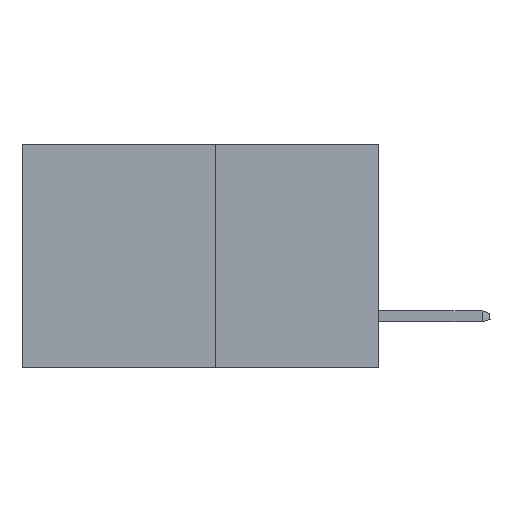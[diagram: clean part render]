
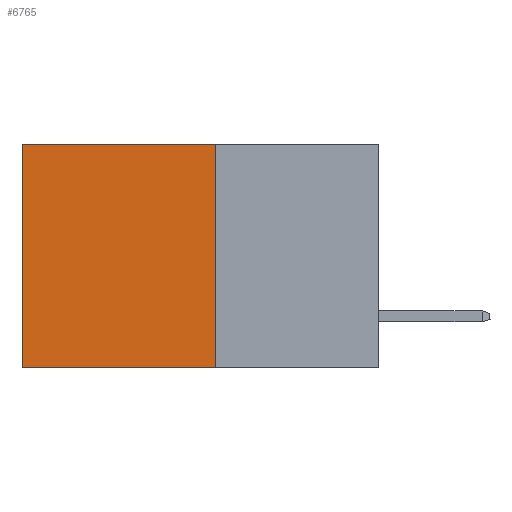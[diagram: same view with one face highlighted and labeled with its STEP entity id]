
A CAD part, left-side view. The second image highlights one B-rep face of the part: STEP entity #6765.
In plain terms, the highlighted planar face has unit normal (-1, 0, 0).
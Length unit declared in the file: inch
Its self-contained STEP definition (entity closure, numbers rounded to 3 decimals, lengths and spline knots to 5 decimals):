
#218 = ORIENTED_EDGE ( 'NONE', *, *, #3542, .T. ) ;
#1036 = LINE ( 'NONE', #17125, #4807 ) ;
#1118 = VERTEX_POINT ( 'NONE', #12207 ) ;
#1939 = EDGE_CURVE ( 'NONE', #14651, #1118, #13959, .T. ) ;
#2101 = ORIENTED_EDGE ( 'NONE', *, *, #7734, .T. ) ;
#2367 = DIRECTION ( 'NONE',  ( 0., 0., -1. ) ) ;
#3542 = EDGE_CURVE ( 'NONE', #18680, #8754, #1036, .T. ) ;
#3758 = ORIENTED_EDGE ( 'NONE', *, *, #1939, .F. ) ;
#4144 = VECTOR ( 'NONE', #14980, 39.37008 ) ;
#4807 = VECTOR ( 'NONE', #2367, 39.37008 ) ;
#5263 = CARTESIAN_POINT ( 'NONE',  ( 0.277, 0.27, -0.37 ) ) ;
#5290 = DIRECTION ( 'NONE',  ( 0., 1., 0. ) ) ;
#6765 = ADVANCED_FACE ( 'NONE', ( #9466 ), #14829, .F. ) ;
#7539 = CARTESIAN_POINT ( 'NONE',  ( 0.277, 0.27, -0.37 ) ) ;
#7734 = EDGE_CURVE ( 'NONE', #14651, #18680, #16158, .T. ) ;
#8754 = VERTEX_POINT ( 'NONE', #15843 ) ;
#9466 = FACE_OUTER_BOUND ( 'NONE', #19459, .T. ) ;
#9657 = CARTESIAN_POINT ( 'NONE',  ( 0.277, 0.27, -0.37 ) ) ;
#9986 = EDGE_CURVE ( 'NONE', #1118, #8754, #15811, .T. ) ;
#10418 = DIRECTION ( 'NONE',  ( 0., 0., -1. ) ) ;
#12207 = CARTESIAN_POINT ( 'NONE',  ( 0.277, 0.27, -0.37 ) ) ;
#12299 = VECTOR ( 'NONE', #5290, 39.37008 ) ;
#13959 = LINE ( 'NONE', #9657, #17522 ) ;
#14651 = VERTEX_POINT ( 'NONE', #15709 ) ;
#14829 = PLANE ( 'NONE',  #17242 ) ;
#14980 = DIRECTION ( 'NONE',  ( 0., 1., 0. ) ) ;
#15602 = CARTESIAN_POINT ( 'NONE',  ( 0.277, 0.27, 0. ) ) ;
#15709 = CARTESIAN_POINT ( 'NONE',  ( 0.277, 0.27, 0. ) ) ;
#15811 = LINE ( 'NONE', #5263, #12299 ) ;
#15843 = CARTESIAN_POINT ( 'NONE',  ( 0.277, 0.59, -0.37 ) ) ;
#16158 = LINE ( 'NONE', #15602, #4144 ) ;
#17007 = CARTESIAN_POINT ( 'NONE',  ( 0.277, 0.59, 0. ) ) ;
#17125 = CARTESIAN_POINT ( 'NONE',  ( 0.277, 0.59, -0.37 ) ) ;
#17215 = DIRECTION ( 'NONE',  ( 1., 0., 0. ) ) ;
#17242 = AXIS2_PLACEMENT_3D ( 'NONE', #7539, #17215, #17477 ) ;
#17477 = DIRECTION ( 'NONE',  ( 0., 0., -1. ) ) ;
#17522 = VECTOR ( 'NONE', #10418, 39.37008 ) ;
#17647 = ORIENTED_EDGE ( 'NONE', *, *, #9986, .F. ) ;
#18680 = VERTEX_POINT ( 'NONE', #17007 ) ;
#19459 = EDGE_LOOP ( 'NONE', ( #218, #17647, #3758, #2101 ) ) ;
